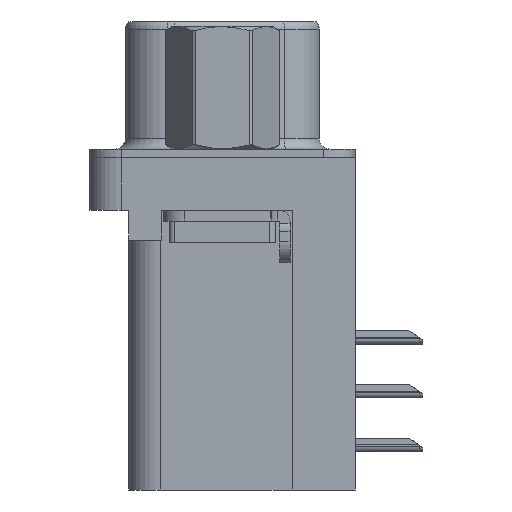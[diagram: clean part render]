
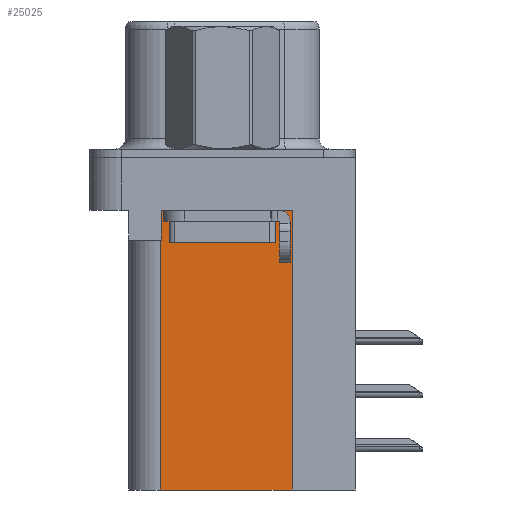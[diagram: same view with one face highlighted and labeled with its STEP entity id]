
A CAD part, left-side view. The second image highlights one B-rep face of the part: STEP entity #25025.
In plain terms, the highlighted planar face has unit normal (-1, 0, 0).
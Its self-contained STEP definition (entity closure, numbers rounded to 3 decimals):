
#556 = ORIENTED_EDGE ( 'NONE', *, *, #12239, .T. ) ;
#882 = VERTEX_POINT ( 'NONE', #22301 ) ;
#2920 = VERTEX_POINT ( 'NONE', #24627 ) ;
#3021 = CARTESIAN_POINT ( 'NONE',  ( 3.7, 2.925, -15.7 ) ) ;
#3324 = CARTESIAN_POINT ( 'NONE',  ( 3.7, -3.295, -15.7 ) ) ;
#3341 = LINE ( 'NONE', #12480, #30097 ) ;
#3690 = VECTOR ( 'NONE', #21250, 1000. ) ;
#3854 = LINE ( 'NONE', #3021, #3690 ) ;
#4398 = CARTESIAN_POINT ( 'NONE',  ( 3.7, 2.895, -2.5 ) ) ;
#4909 = ORIENTED_EDGE ( 'NONE', *, *, #7478, .F. ) ;
#7069 = CARTESIAN_POINT ( 'NONE',  ( 3.7, -3.295, -15.7 ) ) ;
#7478 = EDGE_CURVE ( 'NONE', #13008, #26249, #19181, .T. ) ;
#9089 = VERTEX_POINT ( 'NONE', #4398 ) ;
#9588 = EDGE_CURVE ( 'NONE', #26249, #20576, #3854, .T. ) ;
#9695 = DIRECTION ( 'NONE',  ( 0., 0., 1. ) ) ;
#9788 = CARTESIAN_POINT ( 'NONE',  ( 3.7, 2.925, -15.7 ) ) ;
#10840 = PLANE ( 'NONE',  #26289 ) ;
#10846 = VECTOR ( 'NONE', #18076, 1000. ) ;
#10918 = LINE ( 'NONE', #12845, #10846 ) ;
#12239 = EDGE_CURVE ( 'NONE', #2920, #9089, #10918, .T. ) ;
#12480 = CARTESIAN_POINT ( 'NONE',  ( 3.7, 0., -3.9 ) ) ;
#12845 = CARTESIAN_POINT ( 'NONE',  ( 3.7, -3.295, -2.5 ) ) ;
#13008 = VERTEX_POINT ( 'NONE', #3324 ) ;
#13080 = VECTOR ( 'NONE', #16790, 1000. ) ;
#13372 = DIRECTION ( 'NONE',  ( 0., 0., -1. ) ) ;
#14179 = CARTESIAN_POINT ( 'NONE',  ( 3.7, 2.895, -3.9 ) ) ;
#16039 = VECTOR ( 'NONE', #9695, 1000. ) ;
#16790 = DIRECTION ( 'NONE',  ( 0., 0., -1. ) ) ;
#17837 = EDGE_CURVE ( 'NONE', #13008, #2920, #22965, .T. ) ;
#18076 = DIRECTION ( 'NONE',  ( 0., 1., 0. ) ) ;
#18318 = FACE_OUTER_BOUND ( 'NONE', #25374, .T. ) ;
#19181 = LINE ( 'NONE', #7069, #19204 ) ;
#19204 = VECTOR ( 'NONE', #25094, 1000. ) ;
#19914 = CARTESIAN_POINT ( 'NONE',  ( 3.7, -3.295, -15.7 ) ) ;
#20183 = EDGE_CURVE ( 'NONE', #9089, #882, #33797, .T. ) ;
#20576 = VERTEX_POINT ( 'NONE', #26078 ) ;
#21116 = CARTESIAN_POINT ( 'NONE',  ( 3.7, -3.295, -15.7 ) ) ;
#21250 = DIRECTION ( 'NONE',  ( 0., 0., 1. ) ) ;
#22301 = CARTESIAN_POINT ( 'NONE',  ( 3.7, 2.895, -3.9 ) ) ;
#22965 = LINE ( 'NONE', #19914, #16039 ) ;
#24531 = ORIENTED_EDGE ( 'NONE', *, *, #20183, .T. ) ;
#24627 = CARTESIAN_POINT ( 'NONE',  ( 3.7, -3.295, -2.5 ) ) ;
#25025 = ADVANCED_FACE ( 'NONE', ( #18318 ), #10840, .F. ) ;
#25094 = DIRECTION ( 'NONE',  ( 0., 1., 0. ) ) ;
#25374 = EDGE_LOOP ( 'NONE', ( #556, #24531, #33782, #26228, #4909, #30737 ) ) ;
#25395 = EDGE_CURVE ( 'NONE', #882, #20576, #3341, .T. ) ;
#26078 = CARTESIAN_POINT ( 'NONE',  ( 3.7, 2.925, -3.9 ) ) ;
#26228 = ORIENTED_EDGE ( 'NONE', *, *, #9588, .F. ) ;
#26249 = VERTEX_POINT ( 'NONE', #9788 ) ;
#26289 = AXIS2_PLACEMENT_3D ( 'NONE', #21116, #28967, #13372 ) ;
#28056 = DIRECTION ( 'NONE',  ( 0., 1., 0. ) ) ;
#28967 = DIRECTION ( 'NONE',  ( 1., 0., 0. ) ) ;
#30097 = VECTOR ( 'NONE', #28056, 1000. ) ;
#30737 = ORIENTED_EDGE ( 'NONE', *, *, #17837, .T. ) ;
#33782 = ORIENTED_EDGE ( 'NONE', *, *, #25395, .T. ) ;
#33797 = LINE ( 'NONE', #14179, #13080 ) ;
